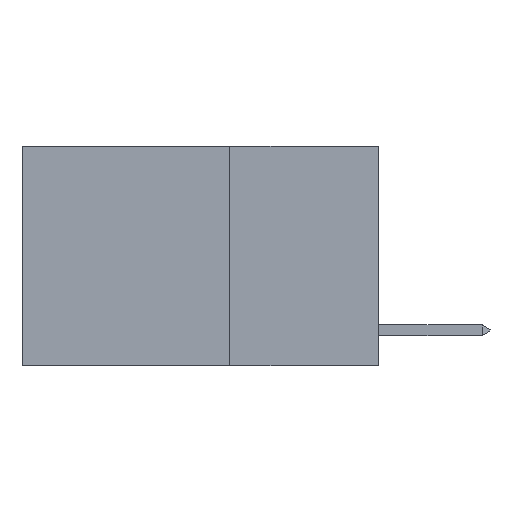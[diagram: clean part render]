
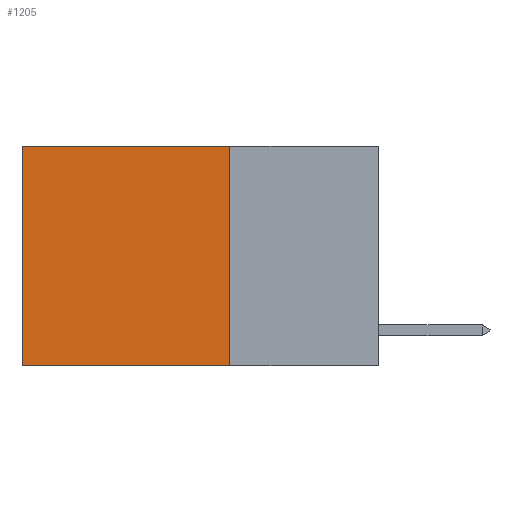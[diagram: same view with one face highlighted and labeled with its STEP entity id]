
A CAD part, left-side view. The second image highlights one B-rep face of the part: STEP entity #1205.
In plain terms, the highlighted planar face has unit normal (-1, 0, 0).
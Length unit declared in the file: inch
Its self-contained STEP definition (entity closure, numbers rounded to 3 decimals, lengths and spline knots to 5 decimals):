
#967 = CARTESIAN_POINT ( 'NONE',  ( 0.2625, 0.25, 0. ) ) ;
#1205 = ADVANCED_FACE ( 'NONE', ( #18971 ), #23008, .F. ) ;
#1272 = DIRECTION ( 'NONE',  ( 0., 0., -1. ) ) ;
#2022 = ORIENTED_EDGE ( 'NONE', *, *, #18721, .T. ) ;
#2141 = CARTESIAN_POINT ( 'NONE',  ( 0.2625, 0.25, -0.37 ) ) ;
#3058 = CARTESIAN_POINT ( 'NONE',  ( 0.2625, 0.6, -0.37 ) ) ;
#3573 = LINE ( 'NONE', #24150, #19428 ) ;
#3831 = CARTESIAN_POINT ( 'NONE',  ( 0.2625, 0.25, -0.37 ) ) ;
#3915 = DIRECTION ( 'NONE',  ( 0., 0., -1. ) ) ;
#3930 = LINE ( 'NONE', #6544, #24448 ) ;
#6075 = VECTOR ( 'NONE', #21758, 39.37008 ) ;
#6257 = CARTESIAN_POINT ( 'NONE',  ( 0.2625, 0.25, 0. ) ) ;
#6544 = CARTESIAN_POINT ( 'NONE',  ( 0.2625, 0.6, 0. ) ) ;
#6949 = ORIENTED_EDGE ( 'NONE', *, *, #13976, .F. ) ;
#9751 = ORIENTED_EDGE ( 'NONE', *, *, #12273, .F. ) ;
#9947 = DIRECTION ( 'NONE',  ( 0., 1., 0. ) ) ;
#10152 = DIRECTION ( 'NONE',  ( 0., 0., -1. ) ) ;
#11600 = VERTEX_POINT ( 'NONE', #3831 ) ;
#12273 = EDGE_CURVE ( 'NONE', #11600, #14300, #22619, .T. ) ;
#13976 = EDGE_CURVE ( 'NONE', #22862, #11600, #3573, .T. ) ;
#14300 = VERTEX_POINT ( 'NONE', #3058 ) ;
#15006 = ORIENTED_EDGE ( 'NONE', *, *, #22372, .T. ) ;
#15013 = CARTESIAN_POINT ( 'NONE',  ( 0.2625, 0.25, 0. ) ) ;
#15567 = EDGE_LOOP ( 'NONE', ( #2022, #9751, #6949, #15006 ) ) ;
#16556 = VERTEX_POINT ( 'NONE', #21861 ) ;
#18721 = EDGE_CURVE ( 'NONE', #16556, #14300, #3930, .T. ) ;
#18971 = FACE_OUTER_BOUND ( 'NONE', #15567, .T. ) ;
#19428 = VECTOR ( 'NONE', #3915, 39.37008 ) ;
#21758 = DIRECTION ( 'NONE',  ( 0., 1., 0. ) ) ;
#21770 = VECTOR ( 'NONE', #9947, 39.37008 ) ;
#21861 = CARTESIAN_POINT ( 'NONE',  ( 0.2625, 0.6, 0. ) ) ;
#22372 = EDGE_CURVE ( 'NONE', #22862, #16556, #22674, .T. ) ;
#22619 = LINE ( 'NONE', #2141, #6075 ) ;
#22674 = LINE ( 'NONE', #6257, #21770 ) ;
#22862 = VERTEX_POINT ( 'NONE', #967 ) ;
#23008 = PLANE ( 'NONE',  #23498 ) ;
#23498 = AXIS2_PLACEMENT_3D ( 'NONE', #15013, #25066, #1272 ) ;
#24150 = CARTESIAN_POINT ( 'NONE',  ( 0.2625, 0.25, 0. ) ) ;
#24448 = VECTOR ( 'NONE', #10152, 39.37008 ) ;
#25066 = DIRECTION ( 'NONE',  ( 1., 0., 0. ) ) ;
